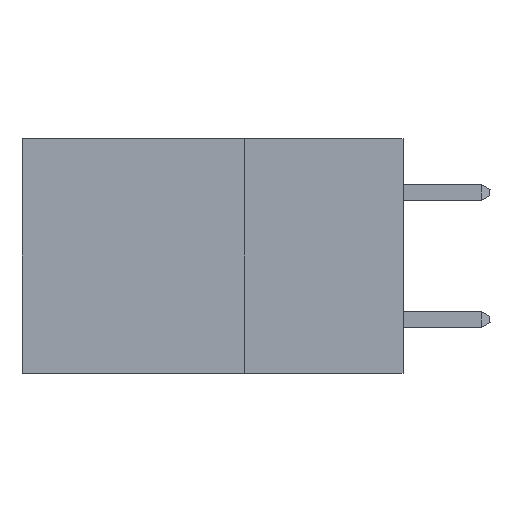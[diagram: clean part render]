
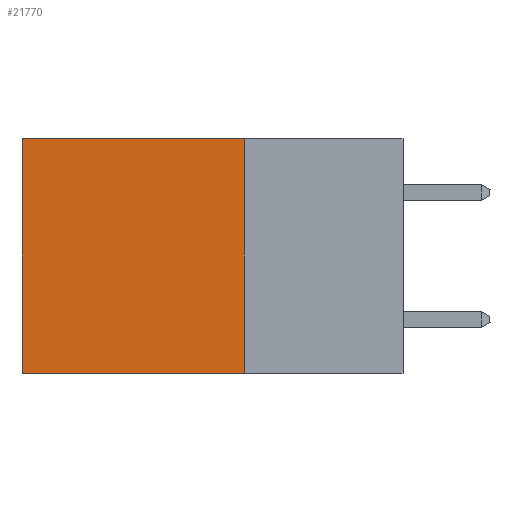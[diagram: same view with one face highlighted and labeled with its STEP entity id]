
A CAD part, left-side view. The second image highlights one B-rep face of the part: STEP entity #21770.
In plain terms, the highlighted planar face has unit normal (-1, 0, 0).
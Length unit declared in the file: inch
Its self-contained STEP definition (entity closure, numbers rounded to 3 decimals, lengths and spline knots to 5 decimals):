
#845 = DIRECTION ( 'NONE',  ( 0., 0., -1. ) ) ;
#4171 = LINE ( 'NONE', #42850, #18056 ) ;
#5448 = EDGE_CURVE ( 'NONE', #35285, #27029, #13894, .T. ) ;
#6244 = EDGE_CURVE ( 'NONE', #28092, #23435, #4171, .T. ) ;
#6918 = LINE ( 'NONE', #31378, #14970 ) ;
#7138 = DIRECTION ( 'NONE',  ( 0., 1., 0. ) ) ;
#8833 = ORIENTED_EDGE ( 'NONE', *, *, #6244, .T. ) ;
#10153 = VECTOR ( 'NONE', #37614, 39.37008 ) ;
#11472 = CARTESIAN_POINT ( 'NONE',  ( 0.2875, 0.25, 0. ) ) ;
#12819 = EDGE_CURVE ( 'NONE', #23435, #27029, #28274, .T. ) ;
#13894 = LINE ( 'NONE', #34096, #28796 ) ;
#14970 = VECTOR ( 'NONE', #845, 39.37008 ) ;
#15840 = ORIENTED_EDGE ( 'NONE', *, *, #12819, .T. ) ;
#17617 = FACE_OUTER_BOUND ( 'NONE', #33256, .T. ) ;
#17677 = CARTESIAN_POINT ( 'NONE',  ( 0.2875, 0.6, 0. ) ) ;
#18056 = VECTOR ( 'NONE', #29087, 39.37008 ) ;
#21770 = ADVANCED_FACE ( 'NONE', ( #17617 ), #41666, .F. ) ;
#23435 = VERTEX_POINT ( 'NONE', #17677 ) ;
#24014 = ORIENTED_EDGE ( 'NONE', *, *, #5448, .F. ) ;
#27029 = VERTEX_POINT ( 'NONE', #33247 ) ;
#28092 = VERTEX_POINT ( 'NONE', #11472 ) ;
#28274 = LINE ( 'NONE', #30957, #10153 ) ;
#28796 = VECTOR ( 'NONE', #7138, 39.37008 ) ;
#29087 = DIRECTION ( 'NONE',  ( 0., 1., 0. ) ) ;
#29814 = ORIENTED_EDGE ( 'NONE', *, *, #40314, .F. ) ;
#30957 = CARTESIAN_POINT ( 'NONE',  ( 0.2875, 0.6, 0. ) ) ;
#31378 = CARTESIAN_POINT ( 'NONE',  ( 0.2875, 0.25, 0. ) ) ;
#33247 = CARTESIAN_POINT ( 'NONE',  ( 0.2875, 0.6, -0.37 ) ) ;
#33256 = EDGE_LOOP ( 'NONE', ( #15840, #24014, #29814, #8833 ) ) ;
#34096 = CARTESIAN_POINT ( 'NONE',  ( 0.2875, 0.25, -0.37 ) ) ;
#35285 = VERTEX_POINT ( 'NONE', #38698 ) ;
#37614 = DIRECTION ( 'NONE',  ( 0., 0., -1. ) ) ;
#37814 = DIRECTION ( 'NONE',  ( 0., 0., -1. ) ) ;
#38413 = AXIS2_PLACEMENT_3D ( 'NONE', #41219, #41378, #37814 ) ;
#38698 = CARTESIAN_POINT ( 'NONE',  ( 0.2875, 0.25, -0.37 ) ) ;
#40314 = EDGE_CURVE ( 'NONE', #28092, #35285, #6918, .T. ) ;
#41219 = CARTESIAN_POINT ( 'NONE',  ( 0.2875, 0.25, 0. ) ) ;
#41378 = DIRECTION ( 'NONE',  ( 1., 0., 0. ) ) ;
#41666 = PLANE ( 'NONE',  #38413 ) ;
#42850 = CARTESIAN_POINT ( 'NONE',  ( 0.2875, 0.25, 0. ) ) ;
